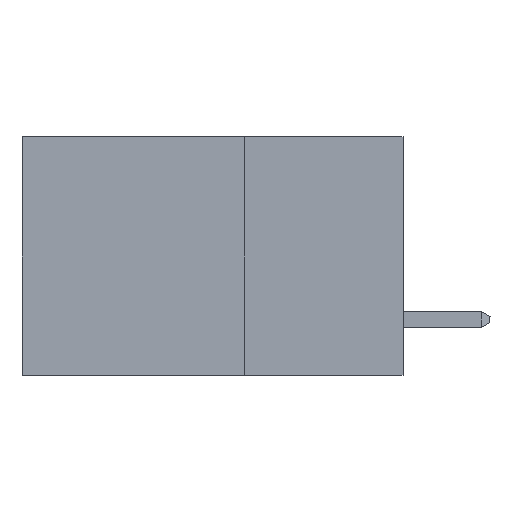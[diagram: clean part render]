
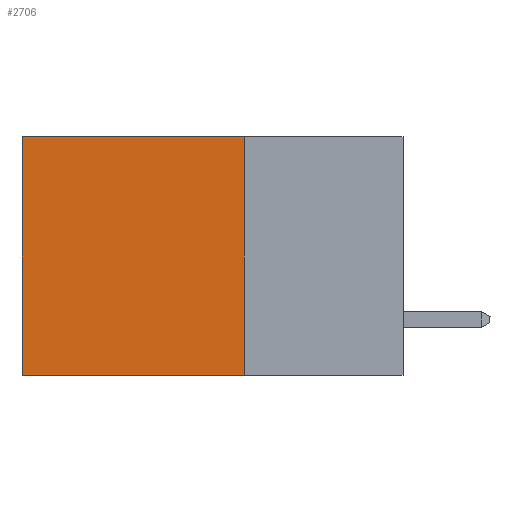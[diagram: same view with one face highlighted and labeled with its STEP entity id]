
A CAD part, left-side view. The second image highlights one B-rep face of the part: STEP entity #2706.
In plain terms, the highlighted planar face has unit normal (-1, 0, 0).
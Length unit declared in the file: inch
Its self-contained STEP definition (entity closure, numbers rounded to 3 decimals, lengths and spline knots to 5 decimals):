
#748 = LINE ( 'NONE', #1151, #7936 ) ;
#891 = ORIENTED_EDGE ( 'NONE', *, *, #5753, .T. ) ;
#952 = VERTEX_POINT ( 'NONE', #6451 ) ;
#989 = EDGE_CURVE ( 'NONE', #7861, #4262, #6871, .T. ) ;
#1052 = FACE_OUTER_BOUND ( 'NONE', #4790, .T. ) ;
#1115 = EDGE_CURVE ( 'NONE', #952, #7861, #4272, .T. ) ;
#1151 = CARTESIAN_POINT ( 'NONE',  ( 0.2875, 0.25, 0. ) ) ;
#1570 = VERTEX_POINT ( 'NONE', #2414 ) ;
#1658 = CARTESIAN_POINT ( 'NONE',  ( 0.2875, 0.6, -0.375 ) ) ;
#1678 = CARTESIAN_POINT ( 'NONE',  ( 0.2875, 0.25, -0.375 ) ) ;
#2141 = VECTOR ( 'NONE', #3764, 39.37008 ) ;
#2414 = CARTESIAN_POINT ( 'NONE',  ( 0.2875, 0.6, 0. ) ) ;
#2440 = PLANE ( 'NONE',  #3346 ) ;
#2603 = ORIENTED_EDGE ( 'NONE', *, *, #1115, .F. ) ;
#2623 = CARTESIAN_POINT ( 'NONE',  ( 0.2875, 0.25, -0.375 ) ) ;
#2706 = ADVANCED_FACE ( 'NONE', ( #1052 ), #2440, .F. ) ;
#2740 = LINE ( 'NONE', #1658, #2141 ) ;
#3252 = VECTOR ( 'NONE', #5230, 39.37008 ) ;
#3346 = AXIS2_PLACEMENT_3D ( 'NONE', #8200, #4394, #5069 ) ;
#3764 = DIRECTION ( 'NONE',  ( 0., 0., -1. ) ) ;
#3941 = CARTESIAN_POINT ( 'NONE',  ( 0.2875, 0.25, -0.375 ) ) ;
#4059 = VECTOR ( 'NONE', #4605, 39.37008 ) ;
#4262 = VERTEX_POINT ( 'NONE', #6213 ) ;
#4272 = LINE ( 'NONE', #3941, #4059 ) ;
#4394 = DIRECTION ( 'NONE',  ( 1., 0., 0. ) ) ;
#4605 = DIRECTION ( 'NONE',  ( 0., 0., -1. ) ) ;
#4790 = EDGE_LOOP ( 'NONE', ( #6777, #6189, #2603, #891 ) ) ;
#4868 = EDGE_CURVE ( 'NONE', #1570, #4262, #2740, .T. ) ;
#5069 = DIRECTION ( 'NONE',  ( 0., 0., -1. ) ) ;
#5230 = DIRECTION ( 'NONE',  ( 0., 1., 0. ) ) ;
#5671 = DIRECTION ( 'NONE',  ( 0., 1., 0. ) ) ;
#5753 = EDGE_CURVE ( 'NONE', #952, #1570, #748, .T. ) ;
#6189 = ORIENTED_EDGE ( 'NONE', *, *, #989, .F. ) ;
#6213 = CARTESIAN_POINT ( 'NONE',  ( 0.2875, 0.6, -0.375 ) ) ;
#6451 = CARTESIAN_POINT ( 'NONE',  ( 0.2875, 0.25, 0. ) ) ;
#6777 = ORIENTED_EDGE ( 'NONE', *, *, #4868, .T. ) ;
#6871 = LINE ( 'NONE', #2623, #3252 ) ;
#7861 = VERTEX_POINT ( 'NONE', #1678 ) ;
#7936 = VECTOR ( 'NONE', #5671, 39.37008 ) ;
#8200 = CARTESIAN_POINT ( 'NONE',  ( 0.2875, 0.25, -0.375 ) ) ;
